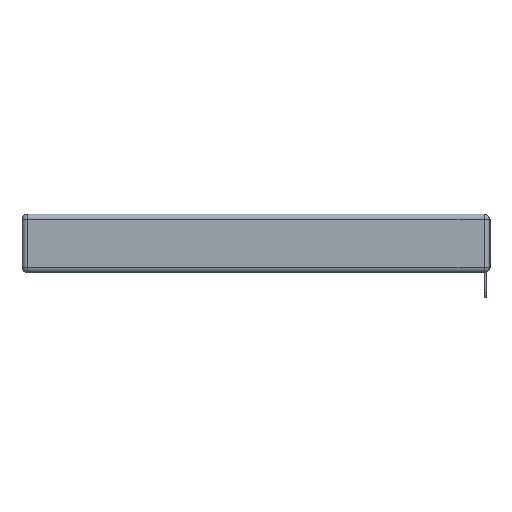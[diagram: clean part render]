
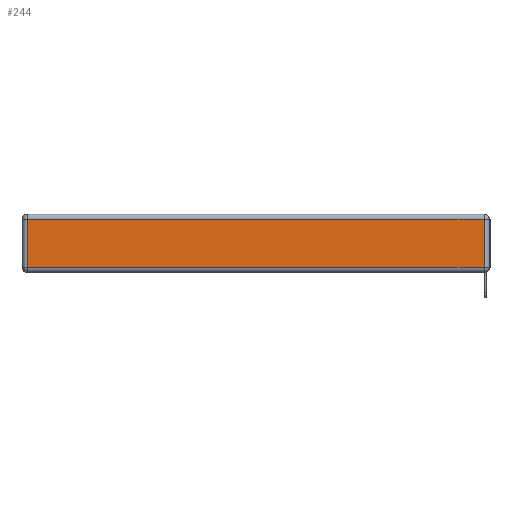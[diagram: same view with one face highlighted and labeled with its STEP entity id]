
A CAD part, left-side view. The second image highlights one B-rep face of the part: STEP entity #244.
In plain terms, the highlighted planar face has unit normal (-1, 0, 0).
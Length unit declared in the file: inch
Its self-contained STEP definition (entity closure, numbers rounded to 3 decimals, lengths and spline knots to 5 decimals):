
#177 = CARTESIAN_POINT ( 'NONE',  ( 0., 0.03, -0.313 ) ) ;
#244 = ADVANCED_FACE ( 'NONE', ( #8665 ), #948, .T. ) ;
#701 = LINE ( 'NONE', #4086, #1957 ) ;
#948 = PLANE ( 'NONE',  #13013 ) ;
#1862 = EDGE_CURVE ( 'NONE', #6354, #10409, #10789, .T. ) ;
#1957 = VECTOR ( 'NONE', #9094, 39.37008 ) ;
#2180 = DIRECTION ( 'NONE',  ( 0., 0., -1. ) ) ;
#2394 = CARTESIAN_POINT ( 'NONE',  ( 0., 2.72, -0.313 ) ) ;
#2946 = CARTESIAN_POINT ( 'NONE',  ( 0., 2.75, -0.03 ) ) ;
#3421 = DIRECTION ( 'NONE',  ( -1., 0., 0. ) ) ;
#3669 = EDGE_LOOP ( 'NONE', ( #5649, #5647, #14949, #12823 ) ) ;
#3807 = VECTOR ( 'NONE', #15288, 39.37008 ) ;
#4086 = CARTESIAN_POINT ( 'NONE',  ( 0., 0., -0.313 ) ) ;
#4571 = CARTESIAN_POINT ( 'NONE',  ( 0., 0., -0.343 ) ) ;
#4761 = VECTOR ( 'NONE', #2180, 39.37008 ) ;
#5003 = VERTEX_POINT ( 'NONE', #2394 ) ;
#5361 = EDGE_CURVE ( 'NONE', #13712, #5003, #8420, .T. ) ;
#5647 = ORIENTED_EDGE ( 'NONE', *, *, #1862, .T. ) ;
#5649 = ORIENTED_EDGE ( 'NONE', *, *, #5729, .T. ) ;
#5729 = EDGE_CURVE ( 'NONE', #5003, #6354, #701, .T. ) ;
#6354 = VERTEX_POINT ( 'NONE', #177 ) ;
#6936 = EDGE_CURVE ( 'NONE', #10409, #13712, #9035, .T. ) ;
#7462 = CARTESIAN_POINT ( 'NONE',  ( 0., 2.72, -0.03 ) ) ;
#8126 = CARTESIAN_POINT ( 'NONE',  ( 0., 0.03, -0.03 ) ) ;
#8420 = LINE ( 'NONE', #13440, #4761 ) ;
#8665 = FACE_OUTER_BOUND ( 'NONE', #3669, .T. ) ;
#9035 = LINE ( 'NONE', #2946, #3807 ) ;
#9094 = DIRECTION ( 'NONE',  ( 0., -1., 0. ) ) ;
#10409 = VERTEX_POINT ( 'NONE', #8126 ) ;
#10789 = LINE ( 'NONE', #14743, #11751 ) ;
#11751 = VECTOR ( 'NONE', #13419, 39.37008 ) ;
#12823 = ORIENTED_EDGE ( 'NONE', *, *, #5361, .T. ) ;
#13013 = AXIS2_PLACEMENT_3D ( 'NONE', #4571, #3421, #14759 ) ;
#13419 = DIRECTION ( 'NONE',  ( 0., 0., 1. ) ) ;
#13440 = CARTESIAN_POINT ( 'NONE',  ( 0., 2.72, -0.343 ) ) ;
#13712 = VERTEX_POINT ( 'NONE', #7462 ) ;
#14743 = CARTESIAN_POINT ( 'NONE',  ( 0., 0.03, -0.343 ) ) ;
#14759 = DIRECTION ( 'NONE',  ( 0., 0., 1. ) ) ;
#14949 = ORIENTED_EDGE ( 'NONE', *, *, #6936, .T. ) ;
#15288 = DIRECTION ( 'NONE',  ( 0., 1., 0. ) ) ;
